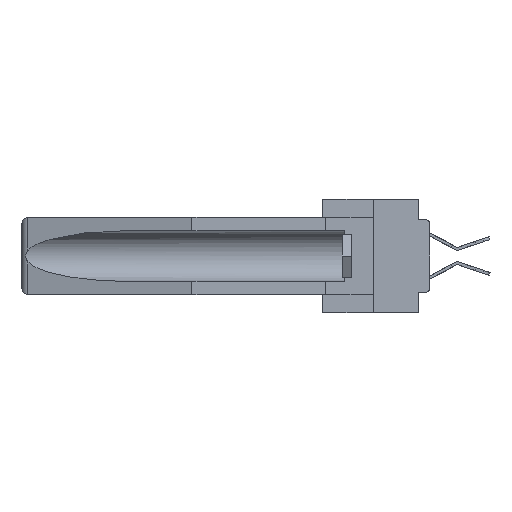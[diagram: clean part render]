
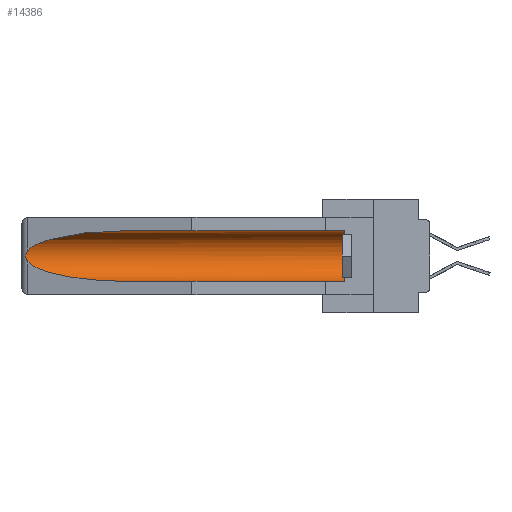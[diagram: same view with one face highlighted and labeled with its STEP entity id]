
A CAD part, left-side view. The second image highlights one B-rep face of the part: STEP entity #14386.
In plain terms, the highlighted cylindrical face has radius 2.857 mm (diameter 5.715 mm), a partial arc.
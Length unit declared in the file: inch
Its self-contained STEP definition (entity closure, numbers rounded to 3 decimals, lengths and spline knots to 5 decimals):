
#98 = CARTESIAN_POINT ( 'NONE',  ( 0.155, -0.30754, -0.1715 ) ) ;
#625 = EDGE_CURVE ( 'NONE', #28050, #34818, #2005, .T. ) ;
#1058 = DIRECTION ( 'NONE',  ( 0., 1., 0. ) ) ;
#1296 = VERTEX_POINT ( 'NONE', #4857 ) ;
#1814 = B_SPLINE_CURVE_WITH_KNOTS ( 'NONE', 3,
 ( #16530, #13442, #21909, #30784, #13809, #30971, #4185, #25354, #28087, #7650 ),
 .UNSPECIFIED., .F., .F.,
 ( 4, 2, 2, 2, 4 ),
 ( 0., 0.00029, 0.00058, 0.00087, 0.00117 ),
 .UNSPECIFIED. ) ;
#2005 =( BOUNDED_CURVE ( )  B_SPLINE_CURVE ( 3, ( #28054, #28238, #24588, #30754 ),
 .UNSPECIFIED., .F., .F. ) 
 B_SPLINE_CURVE_WITH_KNOTS ( ( 4, 4 ),
 ( 0.1948, 1.5708 ),
 .UNSPECIFIED. ) 
 CURVE ( )  GEOMETRIC_REPRESENTATION_ITEM ( )  RATIONAL_B_SPLINE_CURVE ( ( 1., 0.848, 0.848, 1. ) ) 
 REPRESENTATION_ITEM ( '' )  );
#3531 = CARTESIAN_POINT ( 'NONE',  ( 0.21114, 1.30732, -0.059 ) ) ;
#4185 = CARTESIAN_POINT ( 'NONE',  ( 0.2673, 1.53269, -0.17917 ) ) ;
#4857 = CARTESIAN_POINT ( 'NONE',  ( 0.155, 0.126, -0.284 ) ) ;
#6460 = CYLINDRICAL_SURFACE ( 'NONE', #20646, 0.1125 ) ;
#6602 = CARTESIAN_POINT ( 'NONE',  ( 0.26537, 1.52718, -0.14972 ) ) ;
#7650 = CARTESIAN_POINT ( 'NONE',  ( 0.26537, 1.52718, -0.19328 ) ) ;
#7731 = DIRECTION ( 'NONE',  ( 0., -1., 0. ) ) ;
#9279 = CARTESIAN_POINT ( 'NONE',  ( 0.155, -0.30754, -0.284 ) ) ;
#9352 = FACE_OUTER_BOUND ( 'NONE', #37721, .T. ) ;
#9886 =( BOUNDED_CURVE ( )  B_SPLINE_CURVE ( 3, ( #29924, #3531, #24154, #6602 ),
 .UNSPECIFIED., .F., .F. ) 
 B_SPLINE_CURVE_WITH_KNOTS ( ( 4, 4 ),
 ( 4.71239, 6.08839 ),
 .UNSPECIFIED. ) 
 CURVE ( )  GEOMETRIC_REPRESENTATION_ITEM ( )  RATIONAL_B_SPLINE_CURVE ( ( 1., 0.848, 0.848, 1. ) ) 
 REPRESENTATION_ITEM ( '' )  );
#10106 = ORIENTED_EDGE ( 'NONE', *, *, #31920, .T. ) ;
#13156 = CARTESIAN_POINT ( 'NONE',  ( 0.155, 0.126, -0.1715 ) ) ;
#13442 = CARTESIAN_POINT ( 'NONE',  ( 0.26597, 1.52961, -0.15275 ) ) ;
#13809 = CARTESIAN_POINT ( 'NONE',  ( 0.2675, 1.53308, -0.16763 ) ) ;
#14116 = ORIENTED_EDGE ( 'NONE', *, *, #625, .T. ) ;
#14386 = ADVANCED_FACE ( 'NONE', ( #9352 ), #6460, .F. ) ;
#15357 = AXIS2_PLACEMENT_3D ( 'NONE', #13156, #7731, #19482 ) ;
#16273 = EDGE_CURVE ( 'NONE', #17613, #25552, #9886, .T. ) ;
#16447 = EDGE_CURVE ( 'NONE', #25552, #28050, #1814, .T. ) ;
#16530 = CARTESIAN_POINT ( 'NONE',  ( 0.26537, 1.52718, -0.14972 ) ) ;
#17613 = VERTEX_POINT ( 'NONE', #24059 ) ;
#18078 = CARTESIAN_POINT ( 'NONE',  ( 0.155, -0.30754, -0.059 ) ) ;
#18963 = CARTESIAN_POINT ( 'NONE',  ( 0.155, 1.07973, -0.284 ) ) ;
#19482 = DIRECTION ( 'NONE',  ( 0., 0., 1. ) ) ;
#20646 = AXIS2_PLACEMENT_3D ( 'NONE', #98, #24382, #30161 ) ;
#21171 = VERTEX_POINT ( 'NONE', #37131 ) ;
#21909 = CARTESIAN_POINT ( 'NONE',  ( 0.26654, 1.53092, -0.15636 ) ) ;
#23492 = CARTESIAN_POINT ( 'NONE',  ( 0.26537, 1.52718, -0.14972 ) ) ;
#23943 = ORIENTED_EDGE ( 'NONE', *, *, #24225, .T. ) ;
#24059 = CARTESIAN_POINT ( 'NONE',  ( 0.155, 1.07973, -0.059 ) ) ;
#24154 = CARTESIAN_POINT ( 'NONE',  ( 0.25451, 1.48313, -0.09465 ) ) ;
#24225 = EDGE_CURVE ( 'NONE', #21171, #17613, #27845, .T. ) ;
#24382 = DIRECTION ( 'NONE',  ( 0., 1., 0. ) ) ;
#24588 = CARTESIAN_POINT ( 'NONE',  ( 0.21114, 1.30732, -0.284 ) ) ;
#25354 = CARTESIAN_POINT ( 'NONE',  ( 0.26655, 1.53094, -0.18657 ) ) ;
#25552 = VERTEX_POINT ( 'NONE', #23492 ) ;
#26668 = ORIENTED_EDGE ( 'NONE', *, *, #16447, .T. ) ;
#26979 = EDGE_CURVE ( 'NONE', #1296, #34818, #35667, .T. ) ;
#27845 = LINE ( 'NONE', #18078, #31728 ) ;
#28050 = VERTEX_POINT ( 'NONE', #37792 ) ;
#28054 = CARTESIAN_POINT ( 'NONE',  ( 0.26537, 1.52718, -0.19328 ) ) ;
#28087 = CARTESIAN_POINT ( 'NONE',  ( 0.26597, 1.5296, -0.19026 ) ) ;
#28238 = CARTESIAN_POINT ( 'NONE',  ( 0.25451, 1.48313, -0.24835 ) ) ;
#29924 = CARTESIAN_POINT ( 'NONE',  ( 0.155, 1.07973, -0.059 ) ) ;
#30161 = DIRECTION ( 'NONE',  ( 0., 0., 1. ) ) ;
#30754 = CARTESIAN_POINT ( 'NONE',  ( 0.155, 1.07973, -0.284 ) ) ;
#30784 = CARTESIAN_POINT ( 'NONE',  ( 0.2673, 1.5327, -0.16383 ) ) ;
#30971 = CARTESIAN_POINT ( 'NONE',  ( 0.2675, 1.53308, -0.17534 ) ) ;
#31032 = DIRECTION ( 'NONE',  ( 0., 1., 0. ) ) ;
#31728 = VECTOR ( 'NONE', #1058, 39.37008 ) ;
#31920 = EDGE_CURVE ( 'NONE', #1296, #21171, #35017, .T. ) ;
#34339 = ORIENTED_EDGE ( 'NONE', *, *, #26979, .F. ) ;
#34586 = ORIENTED_EDGE ( 'NONE', *, *, #16273, .T. ) ;
#34818 = VERTEX_POINT ( 'NONE', #18963 ) ;
#35017 = CIRCLE ( 'NONE', #15357, 0.1125 ) ;
#35667 = LINE ( 'NONE', #9279, #38012 ) ;
#37131 = CARTESIAN_POINT ( 'NONE',  ( 0.155, 0.126, -0.059 ) ) ;
#37721 = EDGE_LOOP ( 'NONE', ( #34586, #26668, #14116, #34339, #10106, #23943 ) ) ;
#37792 = CARTESIAN_POINT ( 'NONE',  ( 0.26537, 1.52718, -0.19328 ) ) ;
#38012 = VECTOR ( 'NONE', #31032, 39.37008 ) ;
